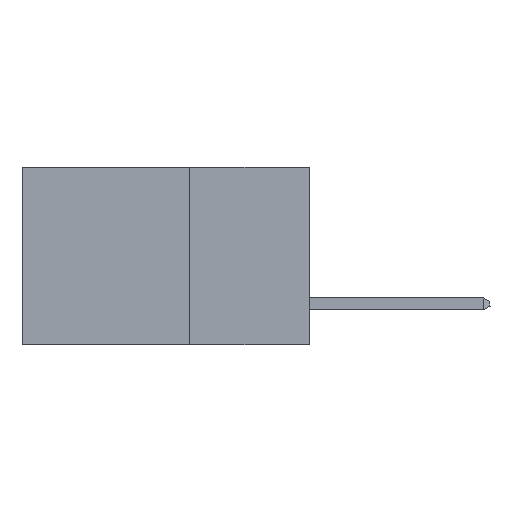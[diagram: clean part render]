
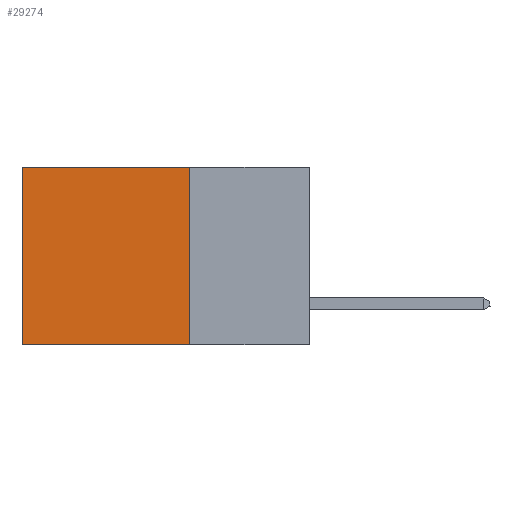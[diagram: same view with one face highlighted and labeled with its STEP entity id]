
A CAD part, left-side view. The second image highlights one B-rep face of the part: STEP entity #29274.
In plain terms, the highlighted planar face has unit normal (-1, 0, 0).
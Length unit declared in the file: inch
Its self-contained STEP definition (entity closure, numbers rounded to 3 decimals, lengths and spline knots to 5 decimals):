
#1772 = DIRECTION ( 'NONE',  ( 0., 1., 0. ) ) ;
#2326 = LINE ( 'NONE', #6319, #36344 ) ;
#2586 = VERTEX_POINT ( 'NONE', #40351 ) ;
#3776 = ORIENTED_EDGE ( 'NONE', *, *, #34921, .T. ) ;
#4984 = ORIENTED_EDGE ( 'NONE', *, *, #5628, .F. ) ;
#5628 = EDGE_CURVE ( 'NONE', #37310, #28581, #13368, .T. ) ;
#6319 = CARTESIAN_POINT ( 'NONE',  ( 0.2875, 0.6, 0. ) ) ;
#9184 = CARTESIAN_POINT ( 'NONE',  ( 0.2875, 0.6, -0.37 ) ) ;
#9228 = FACE_OUTER_BOUND ( 'NONE', #21488, .T. ) ;
#9447 = VERTEX_POINT ( 'NONE', #41660 ) ;
#10385 = DIRECTION ( 'NONE',  ( 0., 0., -1. ) ) ;
#12098 = DIRECTION ( 'NONE',  ( 0., 1., 0. ) ) ;
#13368 = LINE ( 'NONE', #28977, #31459 ) ;
#13706 = PLANE ( 'NONE',  #16388 ) ;
#15032 = EDGE_CURVE ( 'NONE', #2586, #37310, #39045, .T. ) ;
#15181 = CARTESIAN_POINT ( 'NONE',  ( 0.2875, 0.25, 0. ) ) ;
#16388 = AXIS2_PLACEMENT_3D ( 'NONE', #20653, #27300, #10385 ) ;
#16898 = ORIENTED_EDGE ( 'NONE', *, *, #31346, .T. ) ;
#16912 = LINE ( 'NONE', #15181, #25292 ) ;
#18249 = CARTESIAN_POINT ( 'NONE',  ( 0.2875, 0.25, -0.37 ) ) ;
#20118 = ORIENTED_EDGE ( 'NONE', *, *, #15032, .F. ) ;
#20653 = CARTESIAN_POINT ( 'NONE',  ( 0.2875, 0.25, 0. ) ) ;
#21488 = EDGE_LOOP ( 'NONE', ( #16898, #4984, #20118, #3776 ) ) ;
#25292 = VECTOR ( 'NONE', #1772, 39.37008 ) ;
#27300 = DIRECTION ( 'NONE',  ( 1., 0., 0. ) ) ;
#28409 = DIRECTION ( 'NONE',  ( 0., 0., -1. ) ) ;
#28581 = VERTEX_POINT ( 'NONE', #9184 ) ;
#28977 = CARTESIAN_POINT ( 'NONE',  ( 0.2875, 0.25, -0.37 ) ) ;
#29274 = ADVANCED_FACE ( 'NONE', ( #9228 ), #13706, .F. ) ;
#31244 = CARTESIAN_POINT ( 'NONE',  ( 0.2875, 0.25, 0. ) ) ;
#31346 = EDGE_CURVE ( 'NONE', #9447, #28581, #2326, .T. ) ;
#31459 = VECTOR ( 'NONE', #12098, 39.37008 ) ;
#32682 = DIRECTION ( 'NONE',  ( 0., 0., -1. ) ) ;
#34366 = VECTOR ( 'NONE', #28409, 39.37008 ) ;
#34921 = EDGE_CURVE ( 'NONE', #2586, #9447, #16912, .T. ) ;
#36344 = VECTOR ( 'NONE', #32682, 39.37008 ) ;
#37310 = VERTEX_POINT ( 'NONE', #18249 ) ;
#39045 = LINE ( 'NONE', #31244, #34366 ) ;
#40351 = CARTESIAN_POINT ( 'NONE',  ( 0.2875, 0.25, 0. ) ) ;
#41660 = CARTESIAN_POINT ( 'NONE',  ( 0.2875, 0.6, 0. ) ) ;
